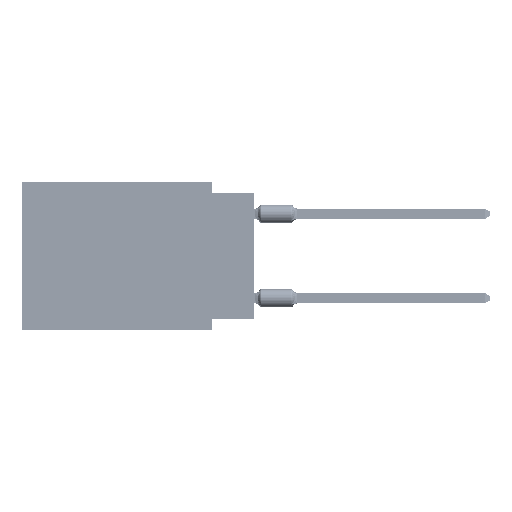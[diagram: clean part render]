
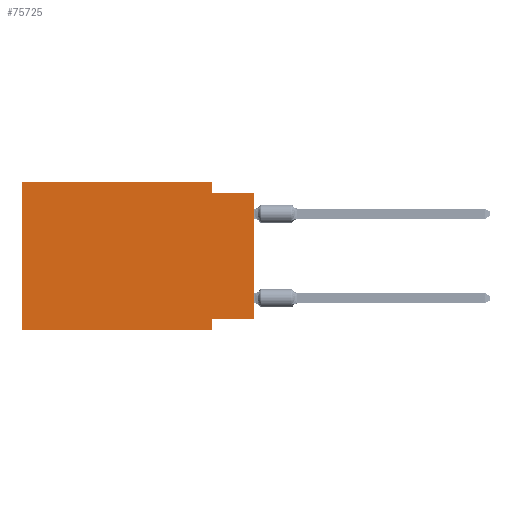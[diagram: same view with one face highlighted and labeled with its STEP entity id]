
A CAD part, left-side view. The second image highlights one B-rep face of the part: STEP entity #75725.
In plain terms, the highlighted planar face has unit normal (-1, 0, 0).
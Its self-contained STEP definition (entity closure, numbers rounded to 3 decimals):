
#1973 = LINE ( 'NONE', #84227, #15167 ) ;
#4164 = EDGE_CURVE ( 'NONE', #85527, #81033, #54479, .T. ) ;
#4999 = CARTESIAN_POINT ( 'NONE',  ( 0., 13.97, 0. ) ) ;
#5692 = ORIENTED_EDGE ( 'NONE', *, *, #78055, .F. ) ;
#7771 = EDGE_CURVE ( 'NONE', #61682, #45243, #41818, .T. ) ;
#8629 = DIRECTION ( 'NONE',  ( 0., 0., -1. ) ) ;
#8995 = LINE ( 'NONE', #24603, #69755 ) ;
#10078 = DIRECTION ( 'NONE',  ( 0., -1., 0. ) ) ;
#12111 = ORIENTED_EDGE ( 'NONE', *, *, #66277, .F. ) ;
#12547 = DIRECTION ( 'NONE',  ( 0., 0., -1. ) ) ;
#14535 = ORIENTED_EDGE ( 'NONE', *, *, #7771, .F. ) ;
#15021 = VECTOR ( 'NONE', #8629, 1000. ) ;
#15167 = VECTOR ( 'NONE', #101382, 1000. ) ;
#17341 = VECTOR ( 'NONE', #46723, 1000. ) ;
#18586 = CARTESIAN_POINT ( 'NONE',  ( 0., 0., -8.255 ) ) ;
#19157 = LINE ( 'NONE', #76677, #91718 ) ;
#19638 = EDGE_CURVE ( 'NONE', #92909, #56798, #98356, .T. ) ;
#23163 = CARTESIAN_POINT ( 'NONE',  ( 0., 2.54, 0. ) ) ;
#24603 = CARTESIAN_POINT ( 'NONE',  ( 0., 0., -8.255 ) ) ;
#32324 = VERTEX_POINT ( 'NONE', #81495 ) ;
#38036 = EDGE_LOOP ( 'NONE', ( #97666, #14535, #12111, #56249, #79182, #72585, #51683, #5692 ) ) ;
#41818 = LINE ( 'NONE', #67615, #72643 ) ;
#45243 = VERTEX_POINT ( 'NONE', #105247 ) ;
#46723 = DIRECTION ( 'NONE',  ( 0., -1., 0. ) ) ;
#46952 = CARTESIAN_POINT ( 'NONE',  ( 0., 13.97, 0. ) ) ;
#51197 = AXIS2_PLACEMENT_3D ( 'NONE', #4999, #69026, #12547 ) ;
#51683 = ORIENTED_EDGE ( 'NONE', *, *, #19638, .F. ) ;
#51932 = DIRECTION ( 'NONE',  ( 0., 0., 1. ) ) ;
#53172 = CARTESIAN_POINT ( 'NONE',  ( 0., 2.54, -8.255 ) ) ;
#53377 = CARTESIAN_POINT ( 'NONE',  ( 0., 2.54, -8.89 ) ) ;
#53392 = FACE_OUTER_BOUND ( 'NONE', #38036, .T. ) ;
#54479 = LINE ( 'NONE', #46952, #78742 ) ;
#56249 = ORIENTED_EDGE ( 'NONE', *, *, #4164, .F. ) ;
#56373 = LINE ( 'NONE', #88635, #17341 ) ;
#56798 = VERTEX_POINT ( 'NONE', #53377 ) ;
#58485 = VERTEX_POINT ( 'NONE', #18586 ) ;
#58560 = CARTESIAN_POINT ( 'NONE',  ( 0., 2.54, -8.89 ) ) ;
#59108 = CARTESIAN_POINT ( 'NONE',  ( 0., 2.54, -0.635 ) ) ;
#61682 = VERTEX_POINT ( 'NONE', #59108 ) ;
#62702 = EDGE_CURVE ( 'NONE', #58485, #45243, #19157, .T. ) ;
#66277 = EDGE_CURVE ( 'NONE', #81033, #61682, #105925, .T. ) ;
#67615 = CARTESIAN_POINT ( 'NONE',  ( 0., 0., -0.635 ) ) ;
#69026 = DIRECTION ( 'NONE',  ( 1., 0., 0. ) ) ;
#69755 = VECTOR ( 'NONE', #83725, 1000. ) ;
#72585 = ORIENTED_EDGE ( 'NONE', *, *, #97099, .T. ) ;
#72643 = VECTOR ( 'NONE', #10078, 1000. ) ;
#75725 = ADVANCED_FACE ( 'NONE', ( #53392 ), #86205, .F. ) ;
#76677 = CARTESIAN_POINT ( 'NONE',  ( 0., 0., 0. ) ) ;
#78055 = EDGE_CURVE ( 'NONE', #58485, #92909, #8995, .T. ) ;
#78742 = VECTOR ( 'NONE', #86767, 1000. ) ;
#79182 = ORIENTED_EDGE ( 'NONE', *, *, #105447, .F. ) ;
#81033 = VERTEX_POINT ( 'NONE', #82220 ) ;
#81495 = CARTESIAN_POINT ( 'NONE',  ( 0., 13.97, -8.89 ) ) ;
#82012 = VECTOR ( 'NONE', #82787, 1000. ) ;
#82220 = CARTESIAN_POINT ( 'NONE',  ( 0., 2.54, 0. ) ) ;
#82787 = DIRECTION ( 'NONE',  ( 0., 0., -1. ) ) ;
#83725 = DIRECTION ( 'NONE',  ( 0., 1., 0. ) ) ;
#84227 = CARTESIAN_POINT ( 'NONE',  ( 0., 13.97, 0. ) ) ;
#85527 = VERTEX_POINT ( 'NONE', #90813 ) ;
#86205 = PLANE ( 'NONE',  #51197 ) ;
#86767 = DIRECTION ( 'NONE',  ( 0., -1., 0. ) ) ;
#88635 = CARTESIAN_POINT ( 'NONE',  ( 0., 13.97, -8.89 ) ) ;
#90813 = CARTESIAN_POINT ( 'NONE',  ( 0., 13.97, 0. ) ) ;
#91718 = VECTOR ( 'NONE', #51932, 1000. ) ;
#92909 = VERTEX_POINT ( 'NONE', #53172 ) ;
#97099 = EDGE_CURVE ( 'NONE', #32324, #56798, #56373, .T. ) ;
#97666 = ORIENTED_EDGE ( 'NONE', *, *, #62702, .T. ) ;
#98356 = LINE ( 'NONE', #58560, #82012 ) ;
#101382 = DIRECTION ( 'NONE',  ( 0., 0., 1. ) ) ;
#105247 = CARTESIAN_POINT ( 'NONE',  ( 0., 0., -0.635 ) ) ;
#105447 = EDGE_CURVE ( 'NONE', #32324, #85527, #1973, .T. ) ;
#105925 = LINE ( 'NONE', #23163, #15021 ) ;
